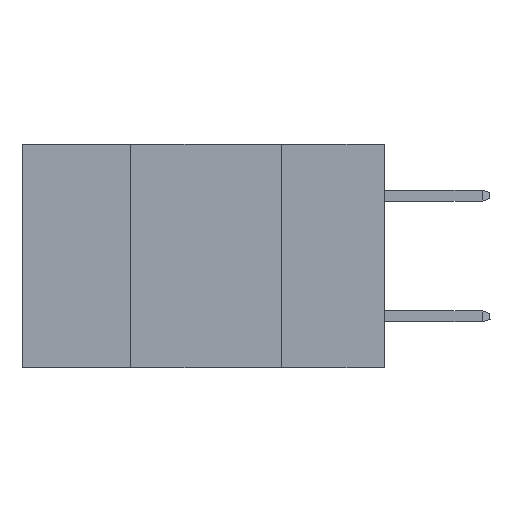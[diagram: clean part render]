
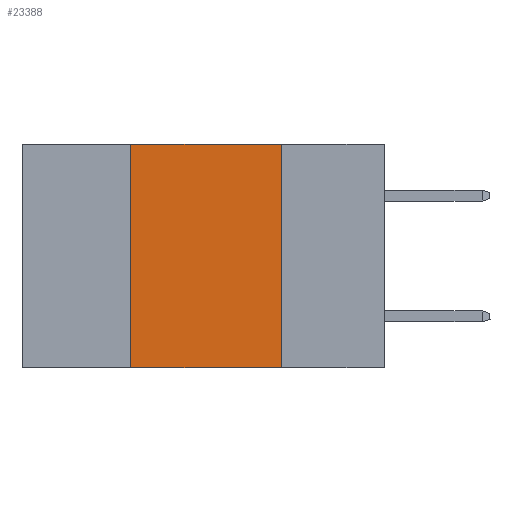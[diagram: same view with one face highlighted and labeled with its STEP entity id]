
A CAD part, left-side view. The second image highlights one B-rep face of the part: STEP entity #23388.
In plain terms, the highlighted planar face has unit normal (-1, 0, 0).
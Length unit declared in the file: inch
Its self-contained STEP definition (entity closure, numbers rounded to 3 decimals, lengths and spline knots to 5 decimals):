
#925 = CARTESIAN_POINT ( 'NONE',  ( 0., 0.42, -0.37 ) ) ;
#2726 = VERTEX_POINT ( 'NONE', #5118 ) ;
#3218 = DIRECTION ( 'NONE',  ( 0., 0., -1. ) ) ;
#4481 = LINE ( 'NONE', #14133, #18468 ) ;
#4994 = CARTESIAN_POINT ( 'NONE',  ( 0., 0.6, 0. ) ) ;
#5091 = VECTOR ( 'NONE', #17213, 39.37008 ) ;
#5118 = CARTESIAN_POINT ( 'NONE',  ( 0., 0.17, -0.37 ) ) ;
#5443 = DIRECTION ( 'NONE',  ( 0., -1., 0. ) ) ;
#5543 = LINE ( 'NONE', #12540, #19518 ) ;
#6714 = ORIENTED_EDGE ( 'NONE', *, *, #19725, .F. ) ;
#7606 = ORIENTED_EDGE ( 'NONE', *, *, #21505, .T. ) ;
#8286 = VERTEX_POINT ( 'NONE', #925 ) ;
#8915 = DIRECTION ( 'NONE',  ( 0., 0., -1. ) ) ;
#9701 = AXIS2_PLACEMENT_3D ( 'NONE', #4994, #14194, #3218 ) ;
#10563 = PLANE ( 'NONE',  #9701 ) ;
#11512 = CARTESIAN_POINT ( 'NONE',  ( 0., 0.17, 0. ) ) ;
#11664 = EDGE_LOOP ( 'NONE', ( #6714, #12238, #13460, #7606 ) ) ;
#12238 = ORIENTED_EDGE ( 'NONE', *, *, #12387, .F. ) ;
#12387 = EDGE_CURVE ( 'NONE', #15455, #22373, #4481, .T. ) ;
#12540 = CARTESIAN_POINT ( 'NONE',  ( 0., 0.17, -0.37 ) ) ;
#12546 = FACE_OUTER_BOUND ( 'NONE', #11664, .T. ) ;
#12810 = CARTESIAN_POINT ( 'NONE',  ( 0., 0.42, 0. ) ) ;
#13460 = ORIENTED_EDGE ( 'NONE', *, *, #17470, .F. ) ;
#14133 = CARTESIAN_POINT ( 'NONE',  ( 0., 0.6, 0. ) ) ;
#14194 = DIRECTION ( 'NONE',  ( 1., 0., 0. ) ) ;
#15179 = LINE ( 'NONE', #20040, #20017 ) ;
#15413 = CARTESIAN_POINT ( 'NONE',  ( 0., 0.42, -0.37 ) ) ;
#15455 = VERTEX_POINT ( 'NONE', #12810 ) ;
#15961 = DIRECTION ( 'NONE',  ( 0., -1., 0. ) ) ;
#17213 = DIRECTION ( 'NONE',  ( 0., 0., 1. ) ) ;
#17470 = EDGE_CURVE ( 'NONE', #8286, #15455, #19640, .T. ) ;
#18468 = VECTOR ( 'NONE', #15961, 39.37008 ) ;
#19518 = VECTOR ( 'NONE', #8915, 39.37008 ) ;
#19640 = LINE ( 'NONE', #15413, #5091 ) ;
#19725 = EDGE_CURVE ( 'NONE', #22373, #2726, #5543, .T. ) ;
#20017 = VECTOR ( 'NONE', #5443, 39.37008 ) ;
#20040 = CARTESIAN_POINT ( 'NONE',  ( 0., 0.6, -0.37 ) ) ;
#21505 = EDGE_CURVE ( 'NONE', #8286, #2726, #15179, .T. ) ;
#22373 = VERTEX_POINT ( 'NONE', #11512 ) ;
#23388 = ADVANCED_FACE ( 'NONE', ( #12546 ), #10563, .F. ) ;
